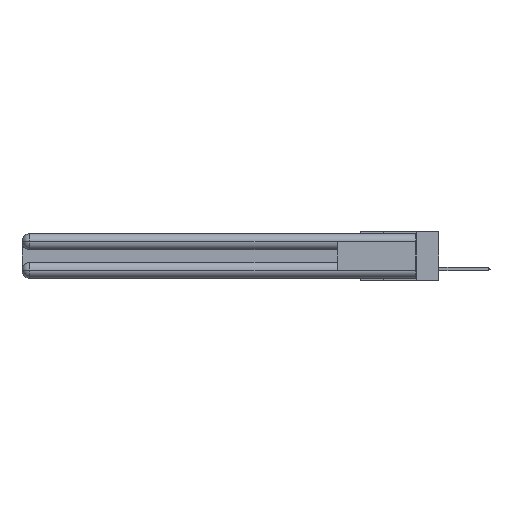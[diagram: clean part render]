
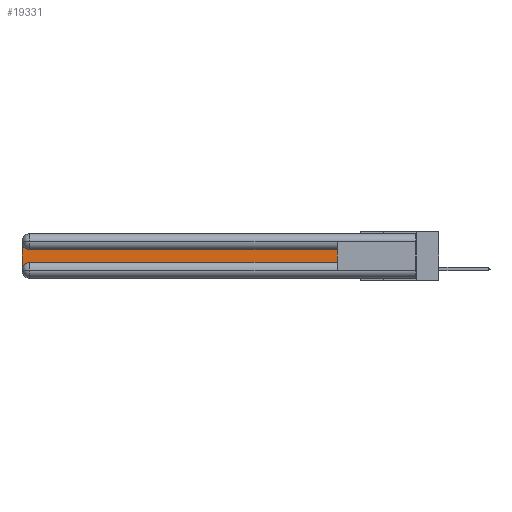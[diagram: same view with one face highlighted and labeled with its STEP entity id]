
A CAD part, left-side view. The second image highlights one B-rep face of the part: STEP entity #19331.
In plain terms, the highlighted planar face has unit normal (-1, 0, 0).
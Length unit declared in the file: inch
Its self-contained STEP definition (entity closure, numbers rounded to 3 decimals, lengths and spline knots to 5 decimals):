
#1040 = CARTESIAN_POINT ( 'NONE',  ( 0.075, 3., -0.2775 ) ) ;
#1260 = VERTEX_POINT ( 'NONE', #6554 ) ;
#1360 = CIRCLE ( 'NONE', #9953, 0.06 ) ;
#1380 = CARTESIAN_POINT ( 'NONE',  ( 0.075, 0.6, -0.2175 ) ) ;
#2187 = ORIENTED_EDGE ( 'NONE', *, *, #17671, .T. ) ;
#2622 = LINE ( 'NONE', #16195, #21642 ) ;
#3065 = CIRCLE ( 'NONE', #24842, 0.06 ) ;
#3995 = EDGE_CURVE ( 'NONE', #31828, #1260, #3065, .T. ) ;
#4057 = VERTEX_POINT ( 'NONE', #1040 ) ;
#5071 = LINE ( 'NONE', #31357, #15953 ) ;
#6385 = DIRECTION ( 'NONE',  ( 0., 0., -1. ) ) ;
#6545 = PLANE ( 'NONE',  #25931 ) ;
#6554 = CARTESIAN_POINT ( 'NONE',  ( 0.075, 3., -0.0625 ) ) ;
#6649 = CARTESIAN_POINT ( 'NONE',  ( 0.075, 3., -0.1225 ) ) ;
#7512 = VERTEX_POINT ( 'NONE', #1380 ) ;
#8187 = CARTESIAN_POINT ( 'NONE',  ( 0.075, 2.94, -0.0625 ) ) ;
#9953 = AXIS2_PLACEMENT_3D ( 'NONE', #20520, #28678, #11189 ) ;
#11189 = DIRECTION ( 'NONE',  ( 0., 0., -1. ) ) ;
#11311 = DIRECTION ( 'NONE',  ( 1., 0., 0. ) ) ;
#11960 = ORIENTED_EDGE ( 'NONE', *, *, #21375, .T. ) ;
#13045 = CARTESIAN_POINT ( 'NONE',  ( 0.075, 0.6, -0.1225 ) ) ;
#13744 = ORIENTED_EDGE ( 'NONE', *, *, #29149, .T. ) ;
#13780 = CARTESIAN_POINT ( 'NONE',  ( 0.075, 0.6, -0.2175 ) ) ;
#15710 = CARTESIAN_POINT ( 'NONE',  ( 0.075, 0.6, -0.1225 ) ) ;
#15953 = VECTOR ( 'NONE', #6385, 39.37008 ) ;
#16159 = VECTOR ( 'NONE', #26085, 39.37008 ) ;
#16195 = CARTESIAN_POINT ( 'NONE',  ( 0.075, 0.6, -0.2175 ) ) ;
#17671 = EDGE_CURVE ( 'NONE', #1260, #4057, #5071, .T. ) ;
#19331 = ADVANCED_FACE ( 'NONE', ( #27513 ), #6545, .F. ) ;
#19874 = EDGE_CURVE ( 'NONE', #7512, #23132, #2622, .T. ) ;
#20022 = VERTEX_POINT ( 'NONE', #24073 ) ;
#20137 = DIRECTION ( 'NONE',  ( 1., 0., 0. ) ) ;
#20520 = CARTESIAN_POINT ( 'NONE',  ( 0.075, 2.94, -0.2775 ) ) ;
#21039 = DIRECTION ( 'NONE',  ( 0., 0., 1. ) ) ;
#21375 = EDGE_CURVE ( 'NONE', #4057, #20022, #1360, .T. ) ;
#21642 = VECTOR ( 'NONE', #21039, 39.37008 ) ;
#22291 = ORIENTED_EDGE ( 'NONE', *, *, #24484, .T. ) ;
#22693 = ORIENTED_EDGE ( 'NONE', *, *, #19874, .T. ) ;
#23132 = VERTEX_POINT ( 'NONE', #13045 ) ;
#24073 = CARTESIAN_POINT ( 'NONE',  ( 0.075, 2.94, -0.2175 ) ) ;
#24484 = EDGE_CURVE ( 'NONE', #20022, #7512, #24974, .T. ) ;
#24842 = AXIS2_PLACEMENT_3D ( 'NONE', #8187, #20137, #28066 ) ;
#24974 = LINE ( 'NONE', #13780, #25355 ) ;
#25355 = VECTOR ( 'NONE', #28659, 39.37008 ) ;
#25931 = AXIS2_PLACEMENT_3D ( 'NONE', #6649, #11311, #30986 ) ;
#25951 = EDGE_LOOP ( 'NONE', ( #13744, #30809, #2187, #11960, #22291, #22693 ) ) ;
#26085 = DIRECTION ( 'NONE',  ( 0., 1., 0. ) ) ;
#27513 = FACE_OUTER_BOUND ( 'NONE', #25951, .T. ) ;
#28066 = DIRECTION ( 'NONE',  ( 0., 0., -1. ) ) ;
#28659 = DIRECTION ( 'NONE',  ( 0., -1., 0. ) ) ;
#28678 = DIRECTION ( 'NONE',  ( 1., 0., 0. ) ) ;
#29149 = EDGE_CURVE ( 'NONE', #23132, #31828, #29357, .T. ) ;
#29357 = LINE ( 'NONE', #15710, #16159 ) ;
#29920 = CARTESIAN_POINT ( 'NONE',  ( 0.075, 2.94, -0.1225 ) ) ;
#30809 = ORIENTED_EDGE ( 'NONE', *, *, #3995, .T. ) ;
#30986 = DIRECTION ( 'NONE',  ( 0., 0., -1. ) ) ;
#31357 = CARTESIAN_POINT ( 'NONE',  ( 0.075, 3., -0.2175 ) ) ;
#31828 = VERTEX_POINT ( 'NONE', #29920 ) ;
